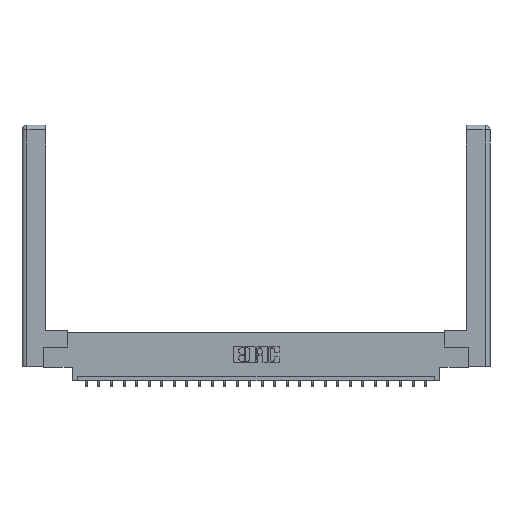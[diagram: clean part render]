
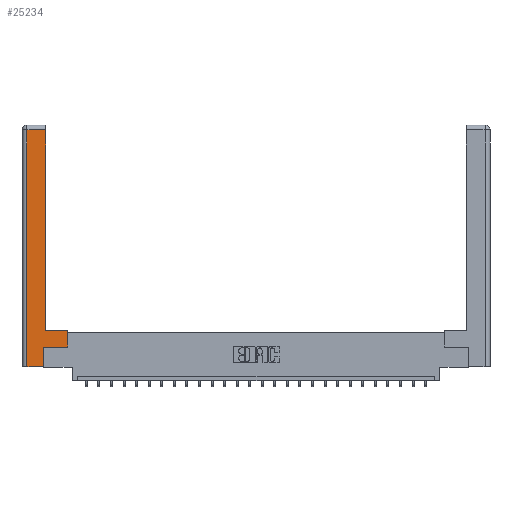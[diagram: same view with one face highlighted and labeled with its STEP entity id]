
A CAD part, top view. The second image highlights one B-rep face of the part: STEP entity #25234.
In plain terms, the highlighted planar face has unit normal (0, 0, 1).
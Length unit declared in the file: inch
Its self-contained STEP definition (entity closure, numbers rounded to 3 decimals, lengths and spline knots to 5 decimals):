
#655 = VERTEX_POINT ( 'NONE', #20838 ) ;
#1148 = DIRECTION ( 'NONE',  ( 0., 1., 0. ) ) ;
#1403 = VERTEX_POINT ( 'NONE', #13809 ) ;
#1633 = CARTESIAN_POINT ( 'NONE',  ( 0.265, 0., 0. ) ) ;
#2144 = CARTESIAN_POINT ( 'NONE',  ( 0.265, 0.245, 0. ) ) ;
#2372 = ORIENTED_EDGE ( 'NONE', *, *, #8418, .T. ) ;
#2466 = LINE ( 'NONE', #16105, #17543 ) ;
#3140 = VECTOR ( 'NONE', #21142, 39.37008 ) ;
#3247 = FACE_OUTER_BOUND ( 'NONE', #22658, .T. ) ;
#4118 = ORIENTED_EDGE ( 'NONE', *, *, #15462, .T. ) ;
#4166 = VECTOR ( 'NONE', #18910, 39.37008 ) ;
#4180 = VERTEX_POINT ( 'NONE', #4477 ) ;
#4187 = LINE ( 'NONE', #19591, #7560 ) ;
#4477 = CARTESIAN_POINT ( 'NONE',  ( 0.565, 0.45, 0. ) ) ;
#4648 = ORIENTED_EDGE ( 'NONE', *, *, #13974, .T. ) ;
#4820 = LINE ( 'NONE', #16302, #12505 ) ;
#4836 = ORIENTED_EDGE ( 'NONE', *, *, #15186, .T. ) ;
#5027 = CARTESIAN_POINT ( 'NONE',  ( 0.565, 0.45, 0. ) ) ;
#6417 = VECTOR ( 'NONE', #13671, 39.37008 ) ;
#6493 = DIRECTION ( 'NONE',  ( 0., -1., 0. ) ) ;
#6862 = CARTESIAN_POINT ( 'NONE',  ( 0., 0., 0. ) ) ;
#7211 = DIRECTION ( 'NONE',  ( -1., 0., 0. ) ) ;
#7560 = VECTOR ( 'NONE', #25441, 39.37008 ) ;
#7956 = CARTESIAN_POINT ( 'NONE',  ( 0.0615, 2.94, 0. ) ) ;
#8059 = ORIENTED_EDGE ( 'NONE', *, *, #10716, .T. ) ;
#8085 = VECTOR ( 'NONE', #1148, 39.37008 ) ;
#8262 = ORIENTED_EDGE ( 'NONE', *, *, #22754, .T. ) ;
#8418 = EDGE_CURVE ( 'NONE', #13563, #1403, #4820, .T. ) ;
#8445 = PLANE ( 'NONE',  #24427 ) ;
#10716 = EDGE_CURVE ( 'NONE', #23260, #4180, #25028, .T. ) ;
#11014 = DIRECTION ( 'NONE',  ( 0., 0., -1. ) ) ;
#11663 = LINE ( 'NONE', #23657, #6417 ) ;
#12505 = VECTOR ( 'NONE', #6493, 39.37008 ) ;
#12794 = EDGE_CURVE ( 'NONE', #20600, #13563, #4187, .T. ) ;
#13431 = CARTESIAN_POINT ( 'NONE',  ( 0.295, 2.94, 0. ) ) ;
#13563 = VERTEX_POINT ( 'NONE', #7956 ) ;
#13671 = DIRECTION ( 'NONE',  ( 0., 1., 0. ) ) ;
#13809 = CARTESIAN_POINT ( 'NONE',  ( 0.0615, 0., 0. ) ) ;
#13974 = EDGE_CURVE ( 'NONE', #21057, #15206, #23247, .T. ) ;
#15186 = EDGE_CURVE ( 'NONE', #1403, #21057, #22526, .T. ) ;
#15206 = VERTEX_POINT ( 'NONE', #2144 ) ;
#15462 = EDGE_CURVE ( 'NONE', #15206, #23260, #20353, .T. ) ;
#16105 = CARTESIAN_POINT ( 'NONE',  ( 0.295, 0.45, 0. ) ) ;
#16302 = CARTESIAN_POINT ( 'NONE',  ( 0.0615, 0., 0. ) ) ;
#16542 = EDGE_CURVE ( 'NONE', #4180, #655, #2466, .T. ) ;
#17093 = CARTESIAN_POINT ( 'NONE',  ( 0.565, 0.245, 0. ) ) ;
#17258 = ORIENTED_EDGE ( 'NONE', *, *, #16542, .T. ) ;
#17543 = VECTOR ( 'NONE', #24218, 39.37008 ) ;
#17613 = VECTOR ( 'NONE', #19440, 39.37008 ) ;
#18910 = DIRECTION ( 'NONE',  ( 0., 1., 0. ) ) ;
#18999 = CARTESIAN_POINT ( 'NONE',  ( 0.265, 0.245, 0. ) ) ;
#19440 = DIRECTION ( 'NONE',  ( 1., 0., 0. ) ) ;
#19591 = CARTESIAN_POINT ( 'NONE',  ( 0.0615, 2.94, 0. ) ) ;
#20353 = LINE ( 'NONE', #21059, #3140 ) ;
#20600 = VERTEX_POINT ( 'NONE', #13431 ) ;
#20838 = CARTESIAN_POINT ( 'NONE',  ( 0.295, 0.45, 0. ) ) ;
#21057 = VERTEX_POINT ( 'NONE', #22354 ) ;
#21059 = CARTESIAN_POINT ( 'NONE',  ( 0.565, 0.245, 0. ) ) ;
#21142 = DIRECTION ( 'NONE',  ( 1., 0., 0. ) ) ;
#22354 = CARTESIAN_POINT ( 'NONE',  ( 0.265, 0., 0. ) ) ;
#22526 = LINE ( 'NONE', #1633, #17613 ) ;
#22658 = EDGE_LOOP ( 'NONE', ( #8262, #24398, #2372, #4836, #4648, #4118, #8059, #17258 ) ) ;
#22754 = EDGE_CURVE ( 'NONE', #655, #20600, #11663, .T. ) ;
#23247 = LINE ( 'NONE', #18999, #4166 ) ;
#23260 = VERTEX_POINT ( 'NONE', #17093 ) ;
#23657 = CARTESIAN_POINT ( 'NONE',  ( 0.295, 3., 0. ) ) ;
#24218 = DIRECTION ( 'NONE',  ( -1., 0., 0. ) ) ;
#24398 = ORIENTED_EDGE ( 'NONE', *, *, #12794, .T. ) ;
#24427 = AXIS2_PLACEMENT_3D ( 'NONE', #6862, #11014, #7211 ) ;
#25028 = LINE ( 'NONE', #5027, #8085 ) ;
#25234 = ADVANCED_FACE ( 'NONE', ( #3247 ), #8445, .F. ) ;
#25441 = DIRECTION ( 'NONE',  ( -1., 0., 0. ) ) ;
